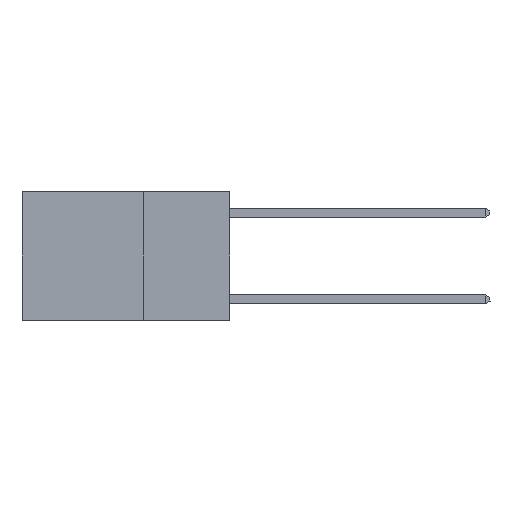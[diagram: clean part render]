
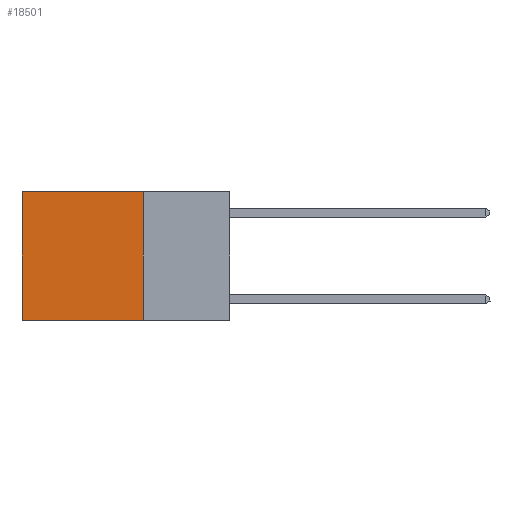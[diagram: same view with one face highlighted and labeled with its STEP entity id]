
A CAD part, left-side view. The second image highlights one B-rep face of the part: STEP entity #18501.
In plain terms, the highlighted planar face has unit normal (-1, 0, 0).
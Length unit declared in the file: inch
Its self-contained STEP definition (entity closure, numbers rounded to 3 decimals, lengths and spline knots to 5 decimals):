
#474 = DIRECTION ( 'NONE',  ( 0., 0., -1. ) ) ;
#607 = CARTESIAN_POINT ( 'NONE',  ( 0.2625, 0.25, 0. ) ) ;
#1069 = VECTOR ( 'NONE', #19143, 39.37008 ) ;
#1115 = ORIENTED_EDGE ( 'NONE', *, *, #4046, .T. ) ;
#1592 = VERTEX_POINT ( 'NONE', #1601 ) ;
#1601 = CARTESIAN_POINT ( 'NONE',  ( 0.2625, 0.6, -0.37 ) ) ;
#2148 = DIRECTION ( 'NONE',  ( 0., 0., -1. ) ) ;
#2322 = ORIENTED_EDGE ( 'NONE', *, *, #9698, .F. ) ;
#3003 = EDGE_CURVE ( 'NONE', #3771, #1592, #12666, .T. ) ;
#3771 = VERTEX_POINT ( 'NONE', #8377 ) ;
#4046 = EDGE_CURVE ( 'NONE', #7734, #3771, #12982, .T. ) ;
#4399 = CARTESIAN_POINT ( 'NONE',  ( 0.2625, 0.25, 0. ) ) ;
#5609 = VERTEX_POINT ( 'NONE', #17151 ) ;
#5663 = LINE ( 'NONE', #16745, #13094 ) ;
#6368 = DIRECTION ( 'NONE',  ( 0., 1., 0. ) ) ;
#6921 = AXIS2_PLACEMENT_3D ( 'NONE', #16721, #7850, #18178 ) ;
#7253 = ORIENTED_EDGE ( 'NONE', *, *, #3003, .T. ) ;
#7734 = VERTEX_POINT ( 'NONE', #607 ) ;
#7850 = DIRECTION ( 'NONE',  ( 1., 0., 0. ) ) ;
#8058 = VECTOR ( 'NONE', #474, 39.37008 ) ;
#8377 = CARTESIAN_POINT ( 'NONE',  ( 0.2625, 0.6, 0. ) ) ;
#9698 = EDGE_CURVE ( 'NONE', #7734, #5609, #12000, .T. ) ;
#10967 = CARTESIAN_POINT ( 'NONE',  ( 0.2625, 0.25, 0. ) ) ;
#11759 = EDGE_LOOP ( 'NONE', ( #7253, #12797, #2322, #1115 ) ) ;
#11807 = EDGE_CURVE ( 'NONE', #5609, #1592, #5663, .T. ) ;
#12000 = LINE ( 'NONE', #10967, #8058 ) ;
#12204 = VECTOR ( 'NONE', #2148, 39.37008 ) ;
#12238 = PLANE ( 'NONE',  #6921 ) ;
#12618 = FACE_OUTER_BOUND ( 'NONE', #11759, .T. ) ;
#12666 = LINE ( 'NONE', #18477, #12204 ) ;
#12797 = ORIENTED_EDGE ( 'NONE', *, *, #11807, .F. ) ;
#12982 = LINE ( 'NONE', #4399, #1069 ) ;
#13094 = VECTOR ( 'NONE', #6368, 39.37008 ) ;
#16721 = CARTESIAN_POINT ( 'NONE',  ( 0.2625, 0.25, 0. ) ) ;
#16745 = CARTESIAN_POINT ( 'NONE',  ( 0.2625, 0.25, -0.37 ) ) ;
#17151 = CARTESIAN_POINT ( 'NONE',  ( 0.2625, 0.25, -0.37 ) ) ;
#18178 = DIRECTION ( 'NONE',  ( 0., 0., -1. ) ) ;
#18477 = CARTESIAN_POINT ( 'NONE',  ( 0.2625, 0.6, 0. ) ) ;
#18501 = ADVANCED_FACE ( 'NONE', ( #12618 ), #12238, .F. ) ;
#19143 = DIRECTION ( 'NONE',  ( 0., 1., 0. ) ) ;
